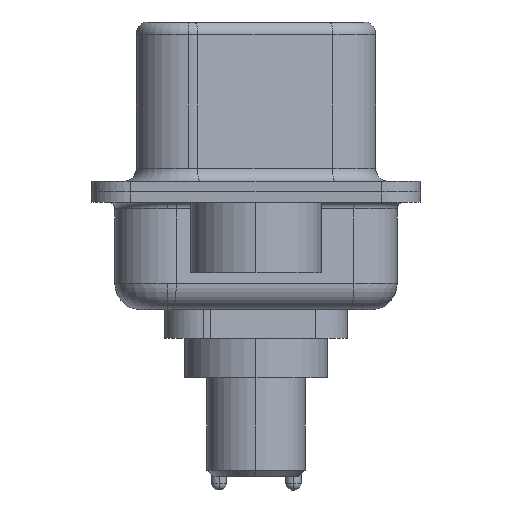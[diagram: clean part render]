
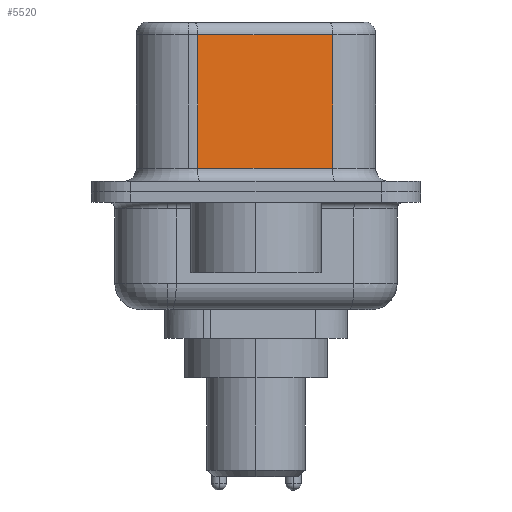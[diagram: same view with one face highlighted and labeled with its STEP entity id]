
A CAD part, left-side view. The second image highlights one B-rep face of the part: STEP entity #5520.
In plain terms, the highlighted planar face has unit normal (-0.985, -0.174, 0).
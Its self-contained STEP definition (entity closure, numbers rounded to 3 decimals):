
#599 = CARTESIAN_POINT ( 'NONE',  ( 4.585, -2.927, 6.02 ) ) ;
#2978 = EDGE_CURVE ( 'NONE', #8575, #9597, #11336, .T. ) ;
#3886 = CARTESIAN_POINT ( 'NONE',  ( 4.585, -2.927, 6.52 ) ) ;
#4582 = PLANE ( 'NONE',  #19628 ) ;
#5168 = DIRECTION ( 'NONE',  ( 0., 0., -1. ) ) ;
#5384 = DIRECTION ( 'NONE',  ( -0.174, 0.985, 0. ) ) ;
#5520 = ADVANCED_FACE ( 'NONE', ( #16046 ), #4582, .F. ) ;
#5540 = DIRECTION ( 'NONE',  ( 0.985, 0.174, 0. ) ) ;
#6401 = LINE ( 'NONE', #17535, #6880 ) ;
#6880 = VECTOR ( 'NONE', #19178, 1000. ) ;
#7157 = CARTESIAN_POINT ( 'NONE',  ( 3.675, 2.233, 0.9 ) ) ;
#7685 = DIRECTION ( 'NONE',  ( 0., 0., -1. ) ) ;
#8017 = VECTOR ( 'NONE', #7685, 1000. ) ;
#8043 = CARTESIAN_POINT ( 'NONE',  ( 3.675, 2.233, 6.02 ) ) ;
#8575 = VERTEX_POINT ( 'NONE', #8043 ) ;
#8866 = ORIENTED_EDGE ( 'NONE', *, *, #13474, .T. ) ;
#9597 = VERTEX_POINT ( 'NONE', #7157 ) ;
#9687 = VERTEX_POINT ( 'NONE', #10637 ) ;
#10637 = CARTESIAN_POINT ( 'NONE',  ( 4.585, -2.927, 6.02 ) ) ;
#10639 = VECTOR ( 'NONE', #5384, 1000. ) ;
#11336 = LINE ( 'NONE', #13968, #8017 ) ;
#11636 = CARTESIAN_POINT ( 'NONE',  ( 4.585, -2.927, 6.52 ) ) ;
#13474 = EDGE_CURVE ( 'NONE', #9687, #8575, #19350, .T. ) ;
#13894 = VECTOR ( 'NONE', #5168, 1000. ) ;
#13968 = CARTESIAN_POINT ( 'NONE',  ( 3.675, 2.233, 6.52 ) ) ;
#14874 = ORIENTED_EDGE ( 'NONE', *, *, #2978, .T. ) ;
#15500 = ORIENTED_EDGE ( 'NONE', *, *, #18168, .F. ) ;
#16046 = FACE_OUTER_BOUND ( 'NONE', #19599, .T. ) ;
#16391 = CARTESIAN_POINT ( 'NONE',  ( 4.585, -2.927, 0.9 ) ) ;
#17535 = CARTESIAN_POINT ( 'NONE',  ( 4.585, -2.927, 0.9 ) ) ;
#17797 = ORIENTED_EDGE ( 'NONE', *, *, #19011, .T. ) ;
#18152 = LINE ( 'NONE', #11636, #13894 ) ;
#18168 = EDGE_CURVE ( 'NONE', #9687, #19942, #18152, .T. ) ;
#19011 = EDGE_CURVE ( 'NONE', #9597, #19942, #6401, .T. ) ;
#19178 = DIRECTION ( 'NONE',  ( 0.174, -0.985, 0. ) ) ;
#19350 = LINE ( 'NONE', #599, #10639 ) ;
#19599 = EDGE_LOOP ( 'NONE', ( #15500, #8866, #14874, #17797 ) ) ;
#19628 = AXIS2_PLACEMENT_3D ( 'NONE', #3886, #5540, #20904 ) ;
#19942 = VERTEX_POINT ( 'NONE', #16391 ) ;
#20904 = DIRECTION ( 'NONE',  ( -0.174, 0.985, 0. ) ) ;
